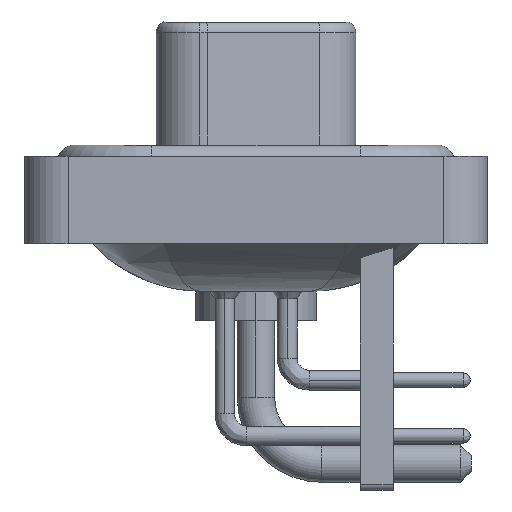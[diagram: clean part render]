
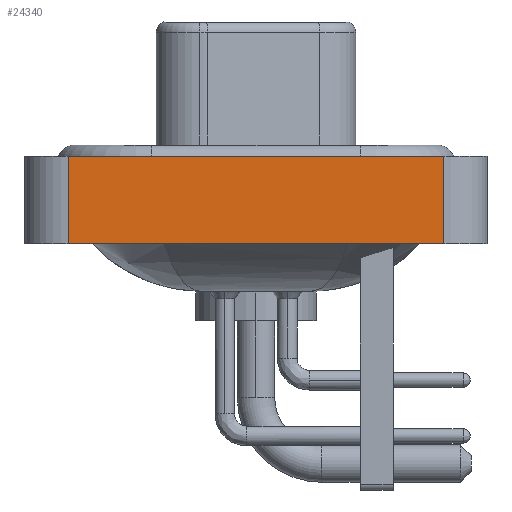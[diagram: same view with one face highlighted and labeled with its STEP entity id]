
A CAD part, left-side view. The second image highlights one B-rep face of the part: STEP entity #24340.
In plain terms, the highlighted planar face has unit normal (-1, 0, 0).
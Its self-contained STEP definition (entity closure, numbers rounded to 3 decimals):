
#123 = LINE ( 'NONE', #25256, #19787 ) ;
#1323 = VECTOR ( 'NONE', #7609, 1000. ) ;
#2954 = VERTEX_POINT ( 'NONE', #24124 ) ;
#3164 = LINE ( 'NONE', #11352, #1323 ) ;
#4373 = EDGE_CURVE ( 'NONE', #23518, #2954, #123, .T. ) ;
#5350 = LINE ( 'NONE', #25768, #18933 ) ;
#5549 = VERTEX_POINT ( 'NONE', #13998 ) ;
#6038 = PLANE ( 'NONE',  #22331 ) ;
#6240 = EDGE_CURVE ( 'NONE', #5549, #23518, #5350, .T. ) ;
#7609 = DIRECTION ( 'NONE',  ( 0., -1., 0. ) ) ;
#8330 = DIRECTION ( 'NONE',  ( 0., 0., 1. ) ) ;
#8549 = LINE ( 'NONE', #16813, #18227 ) ;
#10485 = ORIENTED_EDGE ( 'NONE', *, *, #17873, .F. ) ;
#10589 = EDGE_LOOP ( 'NONE', ( #15181, #21828, #10485, #18880 ) ) ;
#11352 = CARTESIAN_POINT ( 'NONE',  ( -7.3, -8.55, 0.4 ) ) ;
#13323 = CARTESIAN_POINT ( 'NONE',  ( -7.3, -8.55, -3.6 ) ) ;
#13537 = DIRECTION ( 'NONE',  ( 0., -1., 0. ) ) ;
#13998 = CARTESIAN_POINT ( 'NONE',  ( -7.3, 8.55, -3.6 ) ) ;
#14222 = CARTESIAN_POINT ( 'NONE',  ( -7.3, -8.55, -3.6 ) ) ;
#15181 = ORIENTED_EDGE ( 'NONE', *, *, #4373, .T. ) ;
#16285 = FACE_OUTER_BOUND ( 'NONE', #10589, .T. ) ;
#16760 = EDGE_CURVE ( 'NONE', #20946, #2954, #3164, .T. ) ;
#16813 = CARTESIAN_POINT ( 'NONE',  ( -7.3, 8.55, -3.6 ) ) ;
#17873 = EDGE_CURVE ( 'NONE', #5549, #20946, #8549, .T. ) ;
#18227 = VECTOR ( 'NONE', #25077, 1000. ) ;
#18241 = CARTESIAN_POINT ( 'NONE',  ( -7.3, 8.55, 0.4 ) ) ;
#18880 = ORIENTED_EDGE ( 'NONE', *, *, #6240, .T. ) ;
#18933 = VECTOR ( 'NONE', #13537, 1000. ) ;
#19475 = DIRECTION ( 'NONE',  ( -1., 0., 0. ) ) ;
#19787 = VECTOR ( 'NONE', #8330, 1000. ) ;
#20946 = VERTEX_POINT ( 'NONE', #18241 ) ;
#21828 = ORIENTED_EDGE ( 'NONE', *, *, #16760, .F. ) ;
#22331 = AXIS2_PLACEMENT_3D ( 'NONE', #14222, #19475, #23701 ) ;
#23518 = VERTEX_POINT ( 'NONE', #13323 ) ;
#23701 = DIRECTION ( 'NONE',  ( 0., 0., 1. ) ) ;
#24124 = CARTESIAN_POINT ( 'NONE',  ( -7.3, -8.55, 0.4 ) ) ;
#24340 = ADVANCED_FACE ( 'NONE', ( #16285 ), #6038, .T. ) ;
#25077 = DIRECTION ( 'NONE',  ( 0., 0., 1. ) ) ;
#25256 = CARTESIAN_POINT ( 'NONE',  ( -7.3, -8.55, -3.6 ) ) ;
#25768 = CARTESIAN_POINT ( 'NONE',  ( -7.3, -8.55, -3.6 ) ) ;
